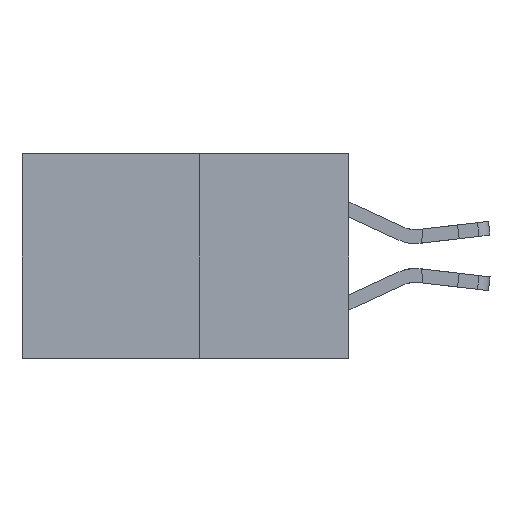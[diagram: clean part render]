
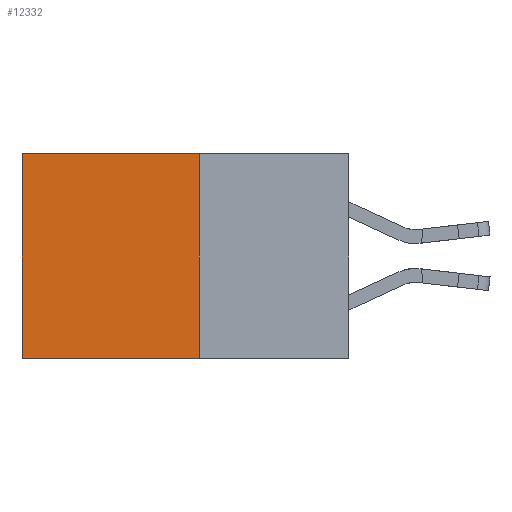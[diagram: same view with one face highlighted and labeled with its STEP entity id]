
A CAD part, left-side view. The second image highlights one B-rep face of the part: STEP entity #12332.
In plain terms, the highlighted planar face has unit normal (-1, 0, 0).
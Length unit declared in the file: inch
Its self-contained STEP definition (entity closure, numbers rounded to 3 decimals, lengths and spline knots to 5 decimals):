
#1524 = VECTOR ( 'NONE', #15723, 39.37008 ) ;
#1586 = CARTESIAN_POINT ( 'NONE',  ( 0.277, 0.27, -0.37 ) ) ;
#2141 = EDGE_CURVE ( 'NONE', #7919, #24591, #9494, .T. ) ;
#2322 = VERTEX_POINT ( 'NONE', #23594 ) ;
#2560 = ORIENTED_EDGE ( 'NONE', *, *, #5816, .T. ) ;
#2796 = VERTEX_POINT ( 'NONE', #19359 ) ;
#3674 = ORIENTED_EDGE ( 'NONE', *, *, #5965, .F. ) ;
#4398 = VECTOR ( 'NONE', #23020, 39.37008 ) ;
#4596 = CARTESIAN_POINT ( 'NONE',  ( 0.277, 0.27, -0.37 ) ) ;
#5634 = ORIENTED_EDGE ( 'NONE', *, *, #14531, .T. ) ;
#5816 = EDGE_CURVE ( 'NONE', #7919, #2796, #17345, .T. ) ;
#5965 = EDGE_CURVE ( 'NONE', #24591, #2322, #23368, .T. ) ;
#7919 = VERTEX_POINT ( 'NONE', #22123 ) ;
#7973 = PLANE ( 'NONE',  #18054 ) ;
#8629 = FACE_OUTER_BOUND ( 'NONE', #21300, .T. ) ;
#9345 = VECTOR ( 'NONE', #23891, 39.37008 ) ;
#9494 = LINE ( 'NONE', #1586, #4398 ) ;
#9913 = DIRECTION ( 'NONE',  ( 1., 0., 0. ) ) ;
#10579 = DIRECTION ( 'NONE',  ( 0., 0., -1. ) ) ;
#11636 = ORIENTED_EDGE ( 'NONE', *, *, #2141, .F. ) ;
#12332 = ADVANCED_FACE ( 'NONE', ( #8629 ), #7973, .F. ) ;
#12375 = LINE ( 'NONE', #23937, #22536 ) ;
#14531 = EDGE_CURVE ( 'NONE', #2796, #2322, #12375, .T. ) ;
#15723 = DIRECTION ( 'NONE',  ( 0., 1., 0. ) ) ;
#17345 = LINE ( 'NONE', #21539, #1524 ) ;
#18054 = AXIS2_PLACEMENT_3D ( 'NONE', #21335, #9913, #23272 ) ;
#19359 = CARTESIAN_POINT ( 'NONE',  ( 0.277, 0.59, 0. ) ) ;
#21300 = EDGE_LOOP ( 'NONE', ( #5634, #3674, #11636, #2560 ) ) ;
#21335 = CARTESIAN_POINT ( 'NONE',  ( 0.277, 0.27, -0.37 ) ) ;
#21539 = CARTESIAN_POINT ( 'NONE',  ( 0.277, 0.27, 0. ) ) ;
#21957 = CARTESIAN_POINT ( 'NONE',  ( 0.277, 0.27, -0.37 ) ) ;
#22123 = CARTESIAN_POINT ( 'NONE',  ( 0.277, 0.27, 0. ) ) ;
#22536 = VECTOR ( 'NONE', #10579, 39.37008 ) ;
#23020 = DIRECTION ( 'NONE',  ( 0., 0., -1. ) ) ;
#23272 = DIRECTION ( 'NONE',  ( 0., 0., -1. ) ) ;
#23368 = LINE ( 'NONE', #21957, #9345 ) ;
#23594 = CARTESIAN_POINT ( 'NONE',  ( 0.277, 0.59, -0.37 ) ) ;
#23891 = DIRECTION ( 'NONE',  ( 0., 1., 0. ) ) ;
#23937 = CARTESIAN_POINT ( 'NONE',  ( 0.277, 0.59, -0.37 ) ) ;
#24591 = VERTEX_POINT ( 'NONE', #4596 ) ;
